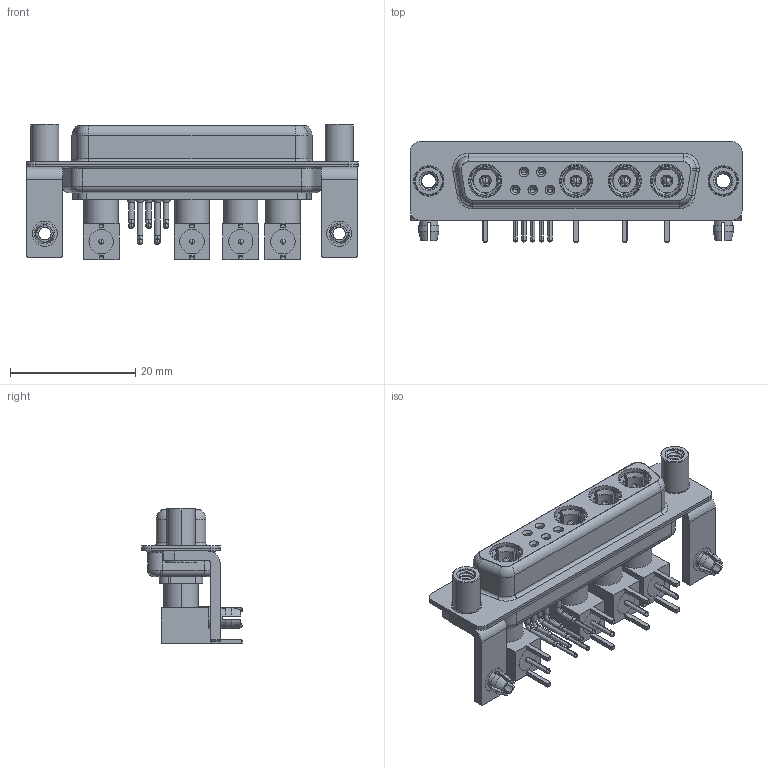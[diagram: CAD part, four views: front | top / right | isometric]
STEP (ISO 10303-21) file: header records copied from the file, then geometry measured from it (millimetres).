
FILE_DESCRIPTION (( 'STEP AP203' ), '1' );
FILE_NAME ('630-9W4-240-7N5.STEP', '2022-06-01T05:37:10', ( '' ), ( '' ), 'SwSTEP 2.0', 'SolidWorks 2020', '' );
FILE_SCHEMA (( 'CONFIG_CONTROL_DESIGN' ));
Length unit declared in the file: millimetre
Products named in the file (19): Pin_RA; Locking Collar; 630Combo Shell Rear_25 Contacts; Co-Ax Plug Assy_RA; Insulator Pin_Straight PC Tail; 630Combo Shell Front_25 Contacts; 630Combo Contact Row 1; 630Combo Contact Row 2; 630Combo Board Lock; Co-Ax Plug_RA PC Tail; 630-9W4-240-7N5; RA Back Shell; 630Combo Stabilizer Bracket; 630Combo Housing_9W4; Insulator RA Pin; 630Combo Threaded Standoff_5
Assembly tree (42 placements, depth 3):
  630-9W4-240-7N5
    630Combo Housing_9W4
    630Combo Shell Front_25 Contacts
    630Combo Shell Rear_25 Contacts
    630Combo Stabilizer Bracket  x2
    630Combo Board Lock  x2
    630Combo Threaded Standoff_5  x2
    Co-Ax Plug Assy_RA
      Co-Ax Plug_RA PC Tail
      Insulator Pin_Straight PC Tail
      Pin_RA
      Locking Collar
      RA Back Shell
      Insulator RA Pin
    Co-Ax Plug Assy_RA
      Co-Ax Plug_RA PC Tail
      Insulator Pin_Straight PC Tail
      Pin_RA
      Locking Collar
      RA Back Shell
      Insulator RA Pin
    Co-Ax Plug Assy_RA
      Co-Ax Plug_RA PC Tail
      Insulator Pin_Straight PC Tail
      Pin_RA
      Locking Collar
      RA Back Shell
      Insulator RA Pin
    Co-Ax Plug Assy_RA
      Co-Ax Plug_RA PC Tail
      Insulator Pin_Straight PC Tail
      Pin_RA
      Locking Collar
      RA Back Shell
      Insulator RA Pin
    630Combo Contact Row 1  x2
    630Combo Contact Row 2  x3
Bounding box: 53.05 x 16 x 21.61 mm (x, y, z)
Volume: 5118.9 mm3; surface area: 12456.5 mm2
Topology: 38 solids, 38 shells, 1396 faces, 3448 edges, 2174 vertices
Faces by surface type: cylinder 604, plane 480, cone 185, torus 81, bspline 30, sphere 16
Entity records: 24635 total; most frequent: CARTESIAN_POINT 5878, DIRECTION 3619, ORIENTED_EDGE 3234, EDGE_CURVE 1617, AXIS2_PLACEMENT_3D 1460, VERTEX_POINT 1031, EDGE_LOOP 760, CIRCLE 759
